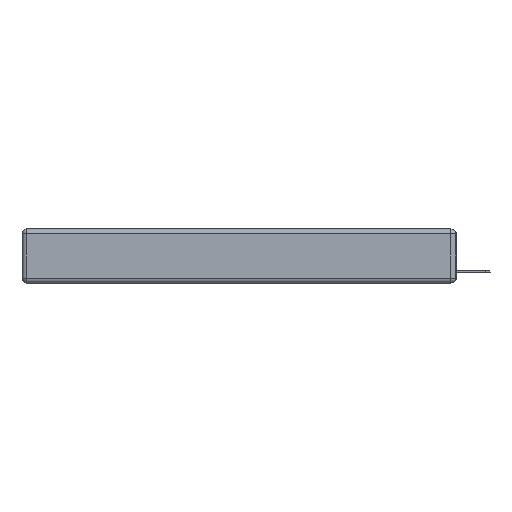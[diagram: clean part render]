
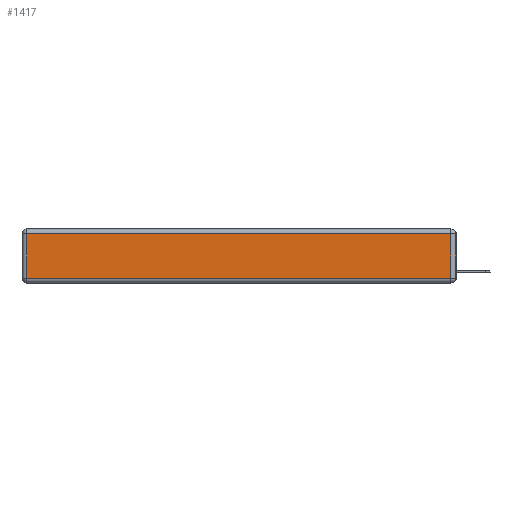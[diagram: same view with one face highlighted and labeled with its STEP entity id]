
A CAD part, left-side view. The second image highlights one B-rep face of the part: STEP entity #1417.
In plain terms, the highlighted planar face has unit normal (-1, 0, 0).
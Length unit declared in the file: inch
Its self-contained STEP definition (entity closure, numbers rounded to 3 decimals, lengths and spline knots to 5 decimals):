
#140 = DIRECTION ( 'NONE',  ( 0., 0., 1. ) ) ;
#506 = EDGE_CURVE ( 'NONE', #11800, #13815, #13718, .T. ) ;
#1328 = CARTESIAN_POINT ( 'NONE',  ( 0., 0.03, -0.03 ) ) ;
#1417 = ADVANCED_FACE ( 'NONE', ( #15622 ), #5610, .T. ) ;
#1814 = LINE ( 'NONE', #11924, #2696 ) ;
#1935 = DIRECTION ( 'NONE',  ( -1., 0., 0. ) ) ;
#2401 = EDGE_CURVE ( 'NONE', #13815, #14621, #1814, .T. ) ;
#2696 = VECTOR ( 'NONE', #5651, 39.37008 ) ;
#4974 = ORIENTED_EDGE ( 'NONE', *, *, #8813, .T. ) ;
#5610 = PLANE ( 'NONE',  #9879 ) ;
#5651 = DIRECTION ( 'NONE',  ( 0., 1., 0. ) ) ;
#6075 = DIRECTION ( 'NONE',  ( 0., -1., 0. ) ) ;
#6902 = DIRECTION ( 'NONE',  ( 0., 0., 1. ) ) ;
#8248 = CARTESIAN_POINT ( 'NONE',  ( 0., 0., -0.313 ) ) ;
#8813 = EDGE_CURVE ( 'NONE', #14487, #11800, #13156, .T. ) ;
#8874 = CARTESIAN_POINT ( 'NONE',  ( 0., 2.72, -0.343 ) ) ;
#9879 = AXIS2_PLACEMENT_3D ( 'NONE', #12041, #1935, #6902 ) ;
#9998 = EDGE_CURVE ( 'NONE', #14621, #14487, #13043, .T. ) ;
#10108 = DIRECTION ( 'NONE',  ( 0., 0., -1. ) ) ;
#10529 = VECTOR ( 'NONE', #140, 39.37008 ) ;
#10568 = ORIENTED_EDGE ( 'NONE', *, *, #9998, .T. ) ;
#10630 = CARTESIAN_POINT ( 'NONE',  ( 0., 2.72, -0.313 ) ) ;
#10709 = CARTESIAN_POINT ( 'NONE',  ( 0., 0.03, -0.313 ) ) ;
#10893 = ORIENTED_EDGE ( 'NONE', *, *, #506, .T. ) ;
#11800 = VERTEX_POINT ( 'NONE', #10709 ) ;
#11924 = CARTESIAN_POINT ( 'NONE',  ( 0., 2.75, -0.03 ) ) ;
#11951 = CARTESIAN_POINT ( 'NONE',  ( 0., 2.72, -0.03 ) ) ;
#12041 = CARTESIAN_POINT ( 'NONE',  ( 0., 0., -0.343 ) ) ;
#12508 = CARTESIAN_POINT ( 'NONE',  ( 0., 0.03, -0.343 ) ) ;
#13043 = LINE ( 'NONE', #8874, #16016 ) ;
#13156 = LINE ( 'NONE', #8248, #14427 ) ;
#13718 = LINE ( 'NONE', #12508, #10529 ) ;
#13815 = VERTEX_POINT ( 'NONE', #1328 ) ;
#14172 = EDGE_LOOP ( 'NONE', ( #4974, #10893, #14846, #10568 ) ) ;
#14427 = VECTOR ( 'NONE', #6075, 39.37008 ) ;
#14487 = VERTEX_POINT ( 'NONE', #10630 ) ;
#14621 = VERTEX_POINT ( 'NONE', #11951 ) ;
#14846 = ORIENTED_EDGE ( 'NONE', *, *, #2401, .T. ) ;
#15622 = FACE_OUTER_BOUND ( 'NONE', #14172, .T. ) ;
#16016 = VECTOR ( 'NONE', #10108, 39.37008 ) ;
